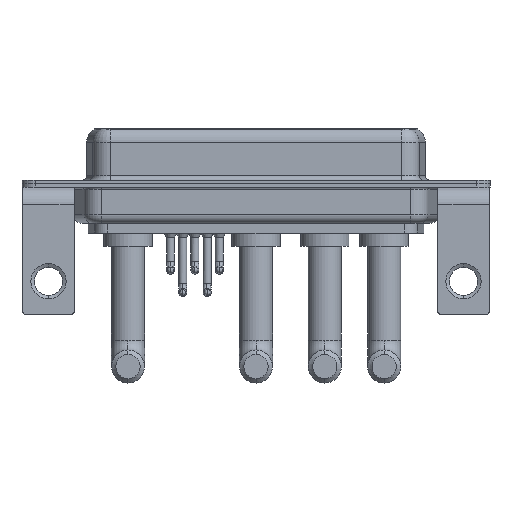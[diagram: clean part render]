
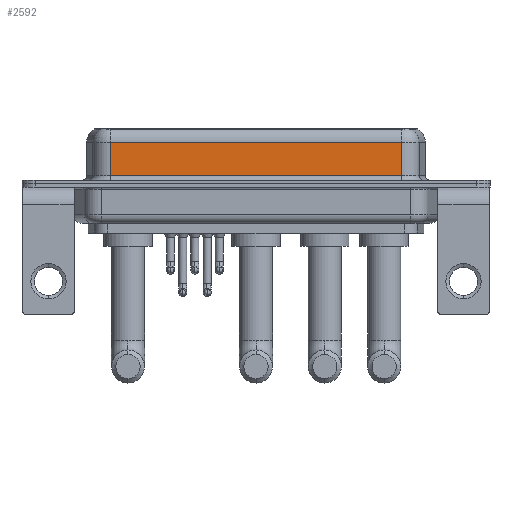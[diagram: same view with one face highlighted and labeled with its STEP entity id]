
A CAD part, front view. The second image highlights one B-rep face of the part: STEP entity #2592.
In plain terms, the highlighted planar face has unit normal (0, -1, 0).
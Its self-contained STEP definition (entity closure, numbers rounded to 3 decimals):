
#70 = EDGE_CURVE ( 'NONE', #14210, #1876, #15434, .T. ) ;
#603 = LINE ( 'NONE', #11751, #9154 ) ;
#844 = ORIENTED_EDGE ( 'NONE', *, *, #1578, .F. ) ;
#1578 = EDGE_CURVE ( 'NONE', #14210, #16909, #603, .T. ) ;
#1848 = DIRECTION ( 'NONE',  ( 0., 1., 0. ) ) ;
#1876 = VERTEX_POINT ( 'NONE', #2601 ) ;
#2100 = EDGE_LOOP ( 'NONE', ( #844, #7504, #17068, #6577 ) ) ;
#2201 = DIRECTION ( 'NONE',  ( 0., 0., 1. ) ) ;
#2592 = ADVANCED_FACE ( 'NONE', ( #10429 ), #14435, .F. ) ;
#2601 = CARTESIAN_POINT ( 'NONE',  ( 7.013, -3.95, 4.65 ) ) ;
#2808 = CARTESIAN_POINT ( 'NONE',  ( 7.013, -3.95, 6.4 ) ) ;
#4165 = LINE ( 'NONE', #2808, #8607 ) ;
#5909 = CARTESIAN_POINT ( 'NONE',  ( 40.037, -3.95, 0.9 ) ) ;
#6577 = ORIENTED_EDGE ( 'NONE', *, *, #8182, .T. ) ;
#7504 = ORIENTED_EDGE ( 'NONE', *, *, #70, .T. ) ;
#8182 = EDGE_CURVE ( 'NONE', #14713, #16909, #17054, .T. ) ;
#8502 = CARTESIAN_POINT ( 'NONE',  ( 40.037, -3.95, 4.65 ) ) ;
#8607 = VECTOR ( 'NONE', #15396, 1000. ) ;
#8897 = AXIS2_PLACEMENT_3D ( 'NONE', #15978, #1848, #2201 ) ;
#8992 = DIRECTION ( 'NONE',  ( 0., 0., -1. ) ) ;
#9154 = VECTOR ( 'NONE', #8992, 1000. ) ;
#10429 = FACE_OUTER_BOUND ( 'NONE', #2100, .T. ) ;
#11751 = CARTESIAN_POINT ( 'NONE',  ( 40.037, -3.95, 6.4 ) ) ;
#12709 = EDGE_CURVE ( 'NONE', #1876, #14713, #4165, .T. ) ;
#13091 = CARTESIAN_POINT ( 'NONE',  ( 40.037, -3.95, 0.9 ) ) ;
#13258 = VECTOR ( 'NONE', #14067, 1000. ) ;
#14067 = DIRECTION ( 'NONE',  ( -1., 0., 0. ) ) ;
#14210 = VERTEX_POINT ( 'NONE', #16666 ) ;
#14435 = PLANE ( 'NONE',  #8897 ) ;
#14713 = VERTEX_POINT ( 'NONE', #16025 ) ;
#15396 = DIRECTION ( 'NONE',  ( 0., 0., -1. ) ) ;
#15434 = LINE ( 'NONE', #8502, #13258 ) ;
#15689 = DIRECTION ( 'NONE',  ( 1., 0., 0. ) ) ;
#15978 = CARTESIAN_POINT ( 'NONE',  ( 40.037, -3.95, 6.4 ) ) ;
#16025 = CARTESIAN_POINT ( 'NONE',  ( 7.013, -3.95, 0.9 ) ) ;
#16610 = VECTOR ( 'NONE', #15689, 1000. ) ;
#16666 = CARTESIAN_POINT ( 'NONE',  ( 40.037, -3.95, 4.65 ) ) ;
#16909 = VERTEX_POINT ( 'NONE', #13091 ) ;
#17054 = LINE ( 'NONE', #5909, #16610 ) ;
#17068 = ORIENTED_EDGE ( 'NONE', *, *, #12709, .T. ) ;
